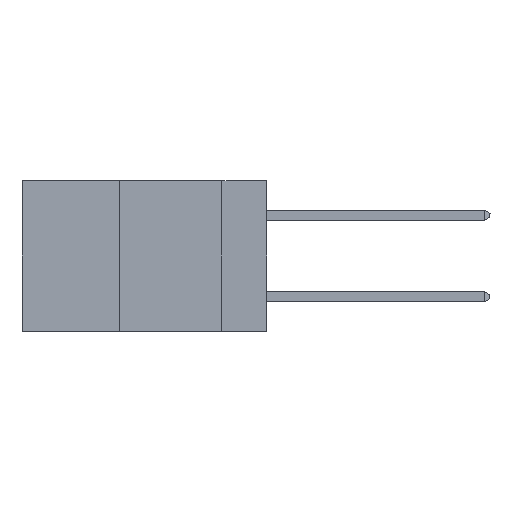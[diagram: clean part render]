
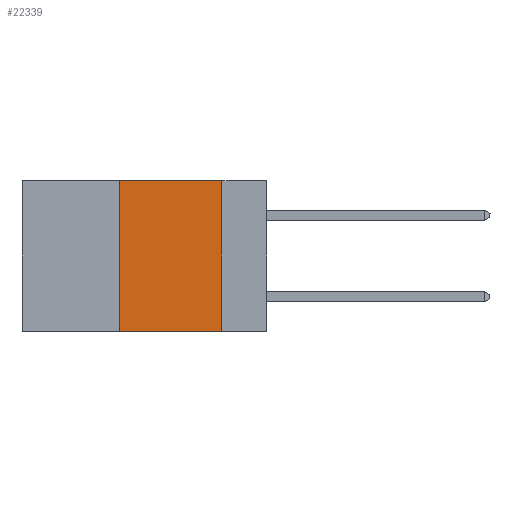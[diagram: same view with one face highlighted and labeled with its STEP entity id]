
A CAD part, left-side view. The second image highlights one B-rep face of the part: STEP entity #22339.
In plain terms, the highlighted planar face has unit normal (-1, 0, 0).
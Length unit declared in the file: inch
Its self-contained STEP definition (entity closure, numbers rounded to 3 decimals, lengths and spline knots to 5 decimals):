
#226 = DIRECTION ( 'NONE',  ( 0., 0., -1. ) ) ;
#290 = ORIENTED_EDGE ( 'NONE', *, *, #17856, .F. ) ;
#401 = PLANE ( 'NONE',  #8357 ) ;
#1171 = CARTESIAN_POINT ( 'NONE',  ( 0., 0.6, 0. ) ) ;
#1674 = LINE ( 'NONE', #20341, #5077 ) ;
#1697 = DIRECTION ( 'NONE',  ( 0., -1., 0. ) ) ;
#3043 = ORIENTED_EDGE ( 'NONE', *, *, #7385, .F. ) ;
#3962 = DIRECTION ( 'NONE',  ( 0., 0., 1. ) ) ;
#5077 = VECTOR ( 'NONE', #3962, 39.37008 ) ;
#6972 = LINE ( 'NONE', #1171, #19420 ) ;
#7385 = EDGE_CURVE ( 'NONE', #24513, #32355, #1674, .T. ) ;
#8158 = CARTESIAN_POINT ( 'NONE',  ( 0., 0.6, 0. ) ) ;
#8357 = AXIS2_PLACEMENT_3D ( 'NONE', #8158, #34636, #226 ) ;
#9258 = VERTEX_POINT ( 'NONE', #29494 ) ;
#9393 = ORIENTED_EDGE ( 'NONE', *, *, #17265, .T. ) ;
#12593 = VECTOR ( 'NONE', #29988, 39.37008 ) ;
#13435 = VERTEX_POINT ( 'NONE', #27683 ) ;
#14250 = LINE ( 'NONE', #24870, #12593 ) ;
#16189 = CARTESIAN_POINT ( 'NONE',  ( 0., 0.36, -0.37 ) ) ;
#17265 = EDGE_CURVE ( 'NONE', #24513, #13435, #14250, .T. ) ;
#17393 = EDGE_LOOP ( 'NONE', ( #31837, #290, #3043, #9393 ) ) ;
#17856 = EDGE_CURVE ( 'NONE', #32355, #9258, #6972, .T. ) ;
#19420 = VECTOR ( 'NONE', #1697, 39.37008 ) ;
#20250 = CARTESIAN_POINT ( 'NONE',  ( 0., 0.36, 0. ) ) ;
#20341 = CARTESIAN_POINT ( 'NONE',  ( 0., 0.36, 0. ) ) ;
#21188 = LINE ( 'NONE', #31963, #33503 ) ;
#21383 = FACE_OUTER_BOUND ( 'NONE', #17393, .T. ) ;
#22339 = ADVANCED_FACE ( 'NONE', ( #21383 ), #401, .F. ) ;
#24513 = VERTEX_POINT ( 'NONE', #16189 ) ;
#24870 = CARTESIAN_POINT ( 'NONE',  ( 0., 0.6, -0.37 ) ) ;
#27683 = CARTESIAN_POINT ( 'NONE',  ( 0., 0.11, -0.37 ) ) ;
#29494 = CARTESIAN_POINT ( 'NONE',  ( 0., 0.11, 0. ) ) ;
#29845 = DIRECTION ( 'NONE',  ( 0., 0., -1. ) ) ;
#29988 = DIRECTION ( 'NONE',  ( 0., -1., 0. ) ) ;
#31837 = ORIENTED_EDGE ( 'NONE', *, *, #33457, .F. ) ;
#31963 = CARTESIAN_POINT ( 'NONE',  ( 0., 0.11, 0. ) ) ;
#32355 = VERTEX_POINT ( 'NONE', #20250 ) ;
#33457 = EDGE_CURVE ( 'NONE', #9258, #13435, #21188, .T. ) ;
#33503 = VECTOR ( 'NONE', #29845, 39.37008 ) ;
#34636 = DIRECTION ( 'NONE',  ( 1., 0., 0. ) ) ;
